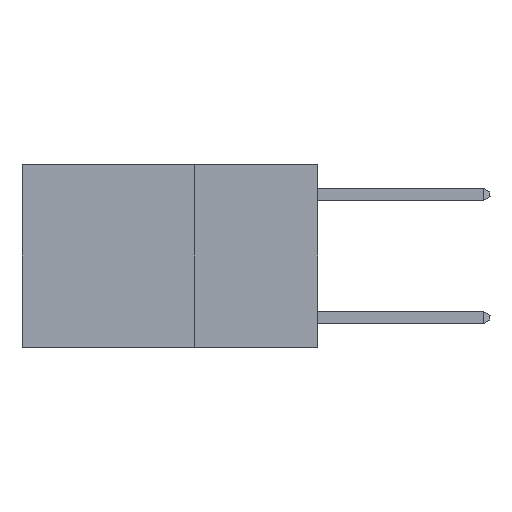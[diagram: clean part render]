
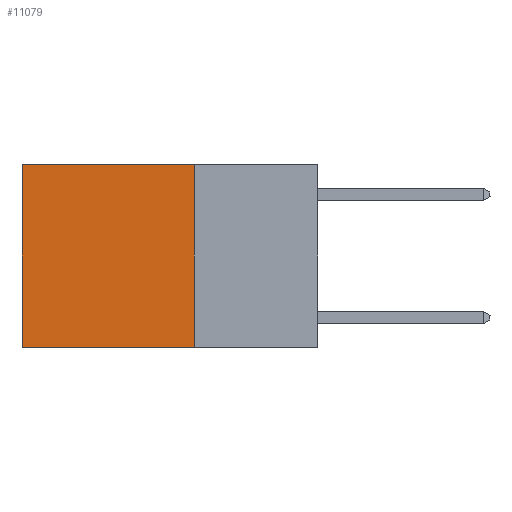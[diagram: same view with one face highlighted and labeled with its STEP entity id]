
A CAD part, left-side view. The second image highlights one B-rep face of the part: STEP entity #11079.
In plain terms, the highlighted planar face has unit normal (-1, 0, 0).
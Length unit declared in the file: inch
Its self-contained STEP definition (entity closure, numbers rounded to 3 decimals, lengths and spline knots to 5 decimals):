
#354 = LINE ( 'NONE', #15056, #23162 ) ;
#474 = VECTOR ( 'NONE', #884, 39.37008 ) ;
#720 = VERTEX_POINT ( 'NONE', #5557 ) ;
#884 = DIRECTION ( 'NONE',  ( 0., 1., 0. ) ) ;
#1697 = DIRECTION ( 'NONE',  ( 0., 1., 0. ) ) ;
#3387 = CARTESIAN_POINT ( 'NONE',  ( 0.2625, 0.25, -0.37 ) ) ;
#3971 = ORIENTED_EDGE ( 'NONE', *, *, #7798, .T. ) ;
#5557 = CARTESIAN_POINT ( 'NONE',  ( 0.2625, 0.6, 0. ) ) ;
#6888 = FACE_OUTER_BOUND ( 'NONE', #18315, .T. ) ;
#7358 = LINE ( 'NONE', #18031, #11992 ) ;
#7472 = DIRECTION ( 'NONE',  ( 0., 0., -1. ) ) ;
#7798 = EDGE_CURVE ( 'NONE', #720, #12171, #10377, .T. ) ;
#8061 = CARTESIAN_POINT ( 'NONE',  ( 0.2625, 0.25, 0. ) ) ;
#8089 = AXIS2_PLACEMENT_3D ( 'NONE', #19746, #17927, #7472 ) ;
#8701 = EDGE_CURVE ( 'NONE', #21442, #20102, #354, .T. ) ;
#9767 = ORIENTED_EDGE ( 'NONE', *, *, #18517, .T. ) ;
#10377 = LINE ( 'NONE', #10840, #10597 ) ;
#10597 = VECTOR ( 'NONE', #18187, 39.37008 ) ;
#10701 = PLANE ( 'NONE',  #8089 ) ;
#10840 = CARTESIAN_POINT ( 'NONE',  ( 0.2625, 0.6, 0. ) ) ;
#10947 = DIRECTION ( 'NONE',  ( 0., 0., -1. ) ) ;
#11079 = ADVANCED_FACE ( 'NONE', ( #6888 ), #10701, .F. ) ;
#11609 = LINE ( 'NONE', #15442, #474 ) ;
#11992 = VECTOR ( 'NONE', #1697, 39.37008 ) ;
#12171 = VERTEX_POINT ( 'NONE', #18056 ) ;
#13373 = EDGE_CURVE ( 'NONE', #20102, #12171, #11609, .T. ) ;
#15056 = CARTESIAN_POINT ( 'NONE',  ( 0.2625, 0.25, 0. ) ) ;
#15442 = CARTESIAN_POINT ( 'NONE',  ( 0.2625, 0.25, -0.37 ) ) ;
#17927 = DIRECTION ( 'NONE',  ( 1., 0., 0. ) ) ;
#18031 = CARTESIAN_POINT ( 'NONE',  ( 0.2625, 0.25, 0. ) ) ;
#18056 = CARTESIAN_POINT ( 'NONE',  ( 0.2625, 0.6, -0.37 ) ) ;
#18187 = DIRECTION ( 'NONE',  ( 0., 0., -1. ) ) ;
#18315 = EDGE_LOOP ( 'NONE', ( #3971, #23406, #21670, #9767 ) ) ;
#18517 = EDGE_CURVE ( 'NONE', #21442, #720, #7358, .T. ) ;
#19746 = CARTESIAN_POINT ( 'NONE',  ( 0.2625, 0.25, 0. ) ) ;
#20102 = VERTEX_POINT ( 'NONE', #3387 ) ;
#21442 = VERTEX_POINT ( 'NONE', #8061 ) ;
#21670 = ORIENTED_EDGE ( 'NONE', *, *, #8701, .F. ) ;
#23162 = VECTOR ( 'NONE', #10947, 39.37008 ) ;
#23406 = ORIENTED_EDGE ( 'NONE', *, *, #13373, .F. ) ;
